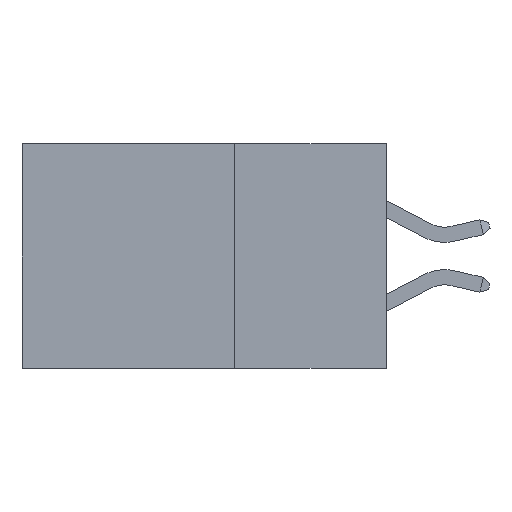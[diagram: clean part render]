
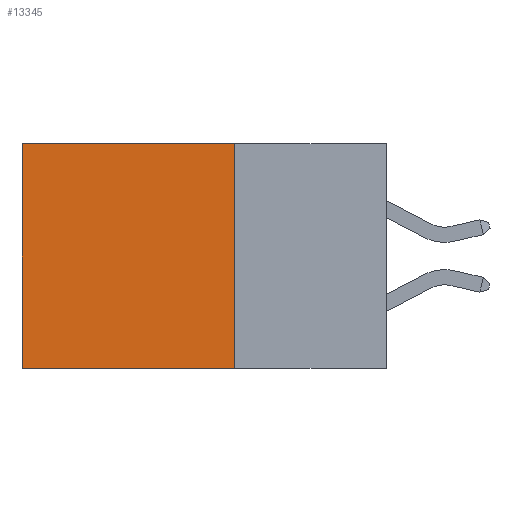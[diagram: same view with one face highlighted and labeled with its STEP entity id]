
A CAD part, left-side view. The second image highlights one B-rep face of the part: STEP entity #13345.
In plain terms, the highlighted planar face has unit normal (-1, 0, 0).
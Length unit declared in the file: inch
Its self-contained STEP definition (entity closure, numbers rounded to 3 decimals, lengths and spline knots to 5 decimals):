
#1822 = CARTESIAN_POINT ( 'NONE',  ( 0.2615, 0.25, -0.37 ) ) ;
#2293 = LINE ( 'NONE', #4217, #8883 ) ;
#2308 = AXIS2_PLACEMENT_3D ( 'NONE', #1822, #21224, #11317 ) ;
#2713 = LINE ( 'NONE', #9289, #5660 ) ;
#2741 = VERTEX_POINT ( 'NONE', #4055 ) ;
#2796 = ORIENTED_EDGE ( 'NONE', *, *, #8559, .F. ) ;
#3418 = VERTEX_POINT ( 'NONE', #14235 ) ;
#4055 = CARTESIAN_POINT ( 'NONE',  ( 0.2615, 0.25, 0. ) ) ;
#4217 = CARTESIAN_POINT ( 'NONE',  ( 0.2615, 0.25, -0.37 ) ) ;
#4742 = DIRECTION ( 'NONE',  ( 0., 0., -1. ) ) ;
#5510 = ORIENTED_EDGE ( 'NONE', *, *, #11704, .T. ) ;
#5660 = VECTOR ( 'NONE', #11011, 39.37008 ) ;
#7139 = DIRECTION ( 'NONE',  ( 0., 1., 0. ) ) ;
#7275 = EDGE_CURVE ( 'NONE', #12917, #3418, #9686, .T. ) ;
#8559 = EDGE_CURVE ( 'NONE', #2741, #16256, #14111, .T. ) ;
#8662 = EDGE_LOOP ( 'NONE', ( #20727, #15521, #2796, #5510 ) ) ;
#8883 = VECTOR ( 'NONE', #7139, 39.37008 ) ;
#9266 = CARTESIAN_POINT ( 'NONE',  ( 0.2615, 0.25, -0.37 ) ) ;
#9289 = CARTESIAN_POINT ( 'NONE',  ( 0.2615, 0.25, 0. ) ) ;
#9686 = LINE ( 'NONE', #13148, #15926 ) ;
#9925 = PLANE ( 'NONE',  #2308 ) ;
#11011 = DIRECTION ( 'NONE',  ( 0., 1., 0. ) ) ;
#11317 = DIRECTION ( 'NONE',  ( 0., 0., -1. ) ) ;
#11704 = EDGE_CURVE ( 'NONE', #2741, #12917, #2713, .T. ) ;
#12917 = VERTEX_POINT ( 'NONE', #16082 ) ;
#13148 = CARTESIAN_POINT ( 'NONE',  ( 0.2615, 0.6, -0.37 ) ) ;
#13155 = FACE_OUTER_BOUND ( 'NONE', #8662, .T. ) ;
#13345 = ADVANCED_FACE ( 'NONE', ( #13155 ), #9925, .F. ) ;
#14076 = CARTESIAN_POINT ( 'NONE',  ( 0.2615, 0.25, -0.37 ) ) ;
#14111 = LINE ( 'NONE', #9266, #16950 ) ;
#14235 = CARTESIAN_POINT ( 'NONE',  ( 0.2615, 0.6, -0.37 ) ) ;
#15254 = EDGE_CURVE ( 'NONE', #16256, #3418, #2293, .T. ) ;
#15521 = ORIENTED_EDGE ( 'NONE', *, *, #15254, .F. ) ;
#15926 = VECTOR ( 'NONE', #4742, 39.37008 ) ;
#16082 = CARTESIAN_POINT ( 'NONE',  ( 0.2615, 0.6, 0. ) ) ;
#16256 = VERTEX_POINT ( 'NONE', #14076 ) ;
#16950 = VECTOR ( 'NONE', #20674, 39.37008 ) ;
#20674 = DIRECTION ( 'NONE',  ( 0., 0., -1. ) ) ;
#20727 = ORIENTED_EDGE ( 'NONE', *, *, #7275, .T. ) ;
#21224 = DIRECTION ( 'NONE',  ( 1., 0., 0. ) ) ;
